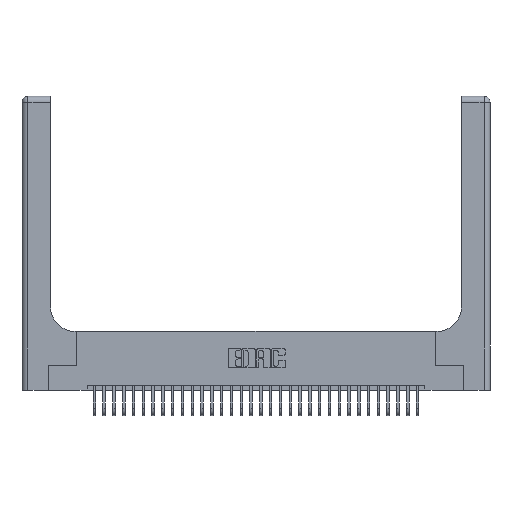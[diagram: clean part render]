
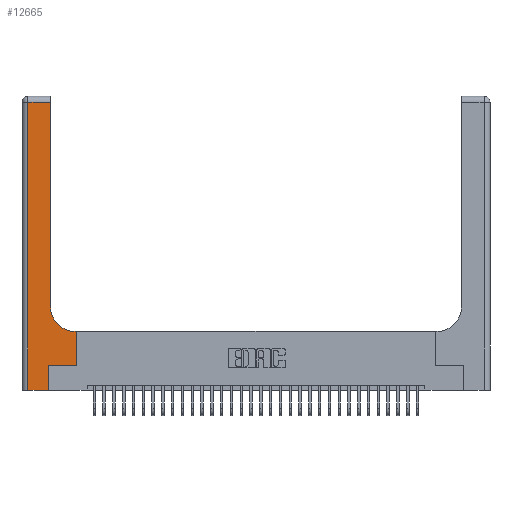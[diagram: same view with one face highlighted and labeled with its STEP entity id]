
A CAD part, top view. The second image highlights one B-rep face of the part: STEP entity #12665.
In plain terms, the highlighted planar face has unit normal (0, 0, 1).
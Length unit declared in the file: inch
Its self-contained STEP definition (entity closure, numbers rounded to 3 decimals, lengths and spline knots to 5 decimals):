
#139 = VECTOR ( 'NONE', #10694, 39.37008 ) ;
#295 = AXIS2_PLACEMENT_3D ( 'NONE', #28786, #29242, #12718 ) ;
#1665 = CIRCLE ( 'NONE', #295, 0.25 ) ;
#2502 = EDGE_CURVE ( 'NONE', #29507, #16562, #2713, .T. ) ;
#2556 = LINE ( 'NONE', #15035, #11718 ) ;
#2631 = CARTESIAN_POINT ( 'NONE',  ( 0.2915, 0.85, 0.37 ) ) ;
#2713 = LINE ( 'NONE', #13136, #12329 ) ;
#2831 = EDGE_CURVE ( 'NONE', #7478, #29507, #13991, .T. ) ;
#3186 = CARTESIAN_POINT ( 'NONE',  ( 0.5585, 0.6, 0.37 ) ) ;
#3542 = PLANE ( 'NONE',  #28229 ) ;
#4376 = CARTESIAN_POINT ( 'NONE',  ( 0.269, 0., 0.37 ) ) ;
#4663 = VERTEX_POINT ( 'NONE', #19848 ) ;
#4830 = EDGE_CURVE ( 'NONE', #21153, #4663, #2556, .T. ) ;
#5303 = ORIENTED_EDGE ( 'NONE', *, *, #2831, .T. ) ;
#5305 = ORIENTED_EDGE ( 'NONE', *, *, #34345, .T. ) ;
#5487 = VECTOR ( 'NONE', #13121, 39.37008 ) ;
#5881 = LINE ( 'NONE', #34510, #5487 ) ;
#6110 = CARTESIAN_POINT ( 'NONE',  ( 0., 3., 0.37 ) ) ;
#6239 = LINE ( 'NONE', #24333, #33411 ) ;
#7478 = VERTEX_POINT ( 'NONE', #8740 ) ;
#8460 = CARTESIAN_POINT ( 'NONE',  ( 0.2915, 2.94, 0.37 ) ) ;
#8740 = CARTESIAN_POINT ( 'NONE',  ( 0.5585, 0.25, 0.37 ) ) ;
#9515 = VECTOR ( 'NONE', #28386, 39.37008 ) ;
#9866 = DIRECTION ( 'NONE',  ( -1., 0., 0. ) ) ;
#10694 = DIRECTION ( 'NONE',  ( 0., -1., 0. ) ) ;
#10813 = CARTESIAN_POINT ( 'NONE',  ( 0.06, 3., 0.37 ) ) ;
#11718 = VECTOR ( 'NONE', #9866, 39.37008 ) ;
#12094 = CARTESIAN_POINT ( 'NONE',  ( 0.06, 0., 0.37 ) ) ;
#12329 = VECTOR ( 'NONE', #23350, 39.37008 ) ;
#12516 = CARTESIAN_POINT ( 'NONE',  ( 0.2915, 3., 0.37 ) ) ;
#12665 = ADVANCED_FACE ( 'NONE', ( #14090 ), #3542, .F. ) ;
#12718 = DIRECTION ( 'NONE',  ( 1., 0., 0. ) ) ;
#12879 = ORIENTED_EDGE ( 'NONE', *, *, #32862, .T. ) ;
#13121 = DIRECTION ( 'NONE',  ( 1., 0., 0. ) ) ;
#13136 = CARTESIAN_POINT ( 'NONE',  ( 0.2915, 0.6, 0.37 ) ) ;
#13817 = DIRECTION ( 'NONE',  ( 1., 0., 0. ) ) ;
#13991 = LINE ( 'NONE', #30551, #26128 ) ;
#14090 = FACE_OUTER_BOUND ( 'NONE', #25451, .T. ) ;
#14556 = DIRECTION ( 'NONE',  ( 0., 1., 0. ) ) ;
#14922 = CARTESIAN_POINT ( 'NONE',  ( 0.269, 0., 0.37 ) ) ;
#15035 = CARTESIAN_POINT ( 'NONE',  ( 0., 2.94, 0.37 ) ) ;
#16562 = VERTEX_POINT ( 'NONE', #21319 ) ;
#17982 = ORIENTED_EDGE ( 'NONE', *, *, #22363, .T. ) ;
#18295 = LINE ( 'NONE', #12516, #31643 ) ;
#19848 = CARTESIAN_POINT ( 'NONE',  ( 0.06, 2.94, 0.37 ) ) ;
#19946 = CARTESIAN_POINT ( 'NONE',  ( 0.269, 0.25, 0.37 ) ) ;
#20483 = ORIENTED_EDGE ( 'NONE', *, *, #32465, .T. ) ;
#20524 = DIRECTION ( 'NONE',  ( 0., 1., 0. ) ) ;
#21153 = VERTEX_POINT ( 'NONE', #8460 ) ;
#21319 = CARTESIAN_POINT ( 'NONE',  ( 0.5415, 0.6, 0.37 ) ) ;
#21683 = ORIENTED_EDGE ( 'NONE', *, *, #4830, .T. ) ;
#22363 = EDGE_CURVE ( 'NONE', #4663, #31535, #22717, .T. ) ;
#22717 = LINE ( 'NONE', #10813, #139 ) ;
#23350 = DIRECTION ( 'NONE',  ( -1., 0., 0. ) ) ;
#23957 = VERTEX_POINT ( 'NONE', #4376 ) ;
#24313 = VERTEX_POINT ( 'NONE', #19946 ) ;
#24333 = CARTESIAN_POINT ( 'NONE',  ( 0.269, 0.25, 0.37 ) ) ;
#25451 = EDGE_LOOP ( 'NONE', ( #34412, #21683, #17982, #5305, #32031, #20483, #5303, #29538, #12879 ) ) ;
#25746 = EDGE_CURVE ( 'NONE', #23957, #24313, #27519, .T. ) ;
#26128 = VECTOR ( 'NONE', #14556, 39.37008 ) ;
#27519 = LINE ( 'NONE', #14922, #9515 ) ;
#28030 = EDGE_CURVE ( 'NONE', #33382, #21153, #18295, .T. ) ;
#28229 = AXIS2_PLACEMENT_3D ( 'NONE', #6110, #29998, #32668 ) ;
#28386 = DIRECTION ( 'NONE',  ( 0., 1., 0. ) ) ;
#28786 = CARTESIAN_POINT ( 'NONE',  ( 0.5415, 0.85, 0.37 ) ) ;
#29242 = DIRECTION ( 'NONE',  ( 0., 0., -1. ) ) ;
#29507 = VERTEX_POINT ( 'NONE', #3186 ) ;
#29538 = ORIENTED_EDGE ( 'NONE', *, *, #2502, .T. ) ;
#29998 = DIRECTION ( 'NONE',  ( 0., 0., -1. ) ) ;
#30551 = CARTESIAN_POINT ( 'NONE',  ( 0.5585, 0.25, 0.37 ) ) ;
#31535 = VERTEX_POINT ( 'NONE', #12094 ) ;
#31643 = VECTOR ( 'NONE', #20524, 39.37008 ) ;
#32031 = ORIENTED_EDGE ( 'NONE', *, *, #25746, .T. ) ;
#32465 = EDGE_CURVE ( 'NONE', #24313, #7478, #6239, .T. ) ;
#32668 = DIRECTION ( 'NONE',  ( -1., 0., 0. ) ) ;
#32862 = EDGE_CURVE ( 'NONE', #16562, #33382, #1665, .T. ) ;
#33382 = VERTEX_POINT ( 'NONE', #2631 ) ;
#33411 = VECTOR ( 'NONE', #13817, 39.37008 ) ;
#34345 = EDGE_CURVE ( 'NONE', #31535, #23957, #5881, .T. ) ;
#34412 = ORIENTED_EDGE ( 'NONE', *, *, #28030, .T. ) ;
#34510 = CARTESIAN_POINT ( 'NONE',  ( 0., 0., 0.37 ) ) ;
